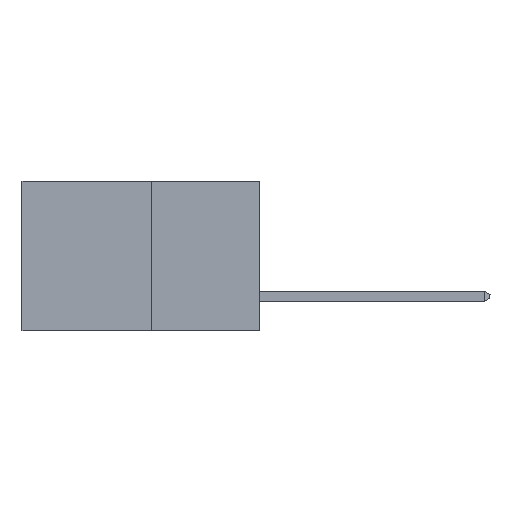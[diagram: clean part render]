
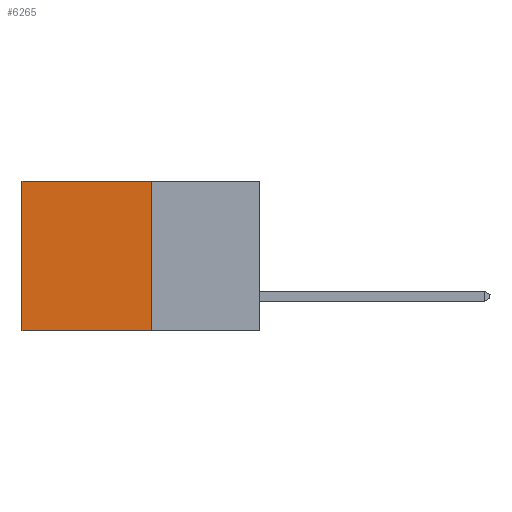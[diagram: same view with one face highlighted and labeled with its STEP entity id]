
A CAD part, left-side view. The second image highlights one B-rep face of the part: STEP entity #6265.
In plain terms, the highlighted planar face has unit normal (-1, 0, 0).
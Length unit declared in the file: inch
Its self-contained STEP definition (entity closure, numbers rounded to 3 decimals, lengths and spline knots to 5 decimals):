
#928 = CARTESIAN_POINT ( 'NONE',  ( 0.277, 0.59, -0.37 ) ) ;
#1916 = CARTESIAN_POINT ( 'NONE',  ( 0.277, 0.59, -0.37 ) ) ;
#2006 = ORIENTED_EDGE ( 'NONE', *, *, #17416, .F. ) ;
#2059 = PLANE ( 'NONE',  #2698 ) ;
#2162 = CARTESIAN_POINT ( 'NONE',  ( 0.277, 0.27, -0.37 ) ) ;
#2698 = AXIS2_PLACEMENT_3D ( 'NONE', #19131, #6349, #21233 ) ;
#3882 = VECTOR ( 'NONE', #4320, 39.37008 ) ;
#3923 = ORIENTED_EDGE ( 'NONE', *, *, #12436, .T. ) ;
#3998 = DIRECTION ( 'NONE',  ( 0., 1., 0. ) ) ;
#4320 = DIRECTION ( 'NONE',  ( 0., 0., -1. ) ) ;
#5439 = VERTEX_POINT ( 'NONE', #22619 ) ;
#6265 = ADVANCED_FACE ( 'NONE', ( #14561 ), #2059, .F. ) ;
#6349 = DIRECTION ( 'NONE',  ( 1., 0., 0. ) ) ;
#7145 = EDGE_LOOP ( 'NONE', ( #3923, #24545, #2006, #20848 ) ) ;
#8177 = CARTESIAN_POINT ( 'NONE',  ( 0.277, 0.27, 0. ) ) ;
#9681 = DIRECTION ( 'NONE',  ( 0., 1., 0. ) ) ;
#11301 = CARTESIAN_POINT ( 'NONE',  ( 0.277, 0.27, -0.37 ) ) ;
#12436 = EDGE_CURVE ( 'NONE', #5439, #22808, #20549, .T. ) ;
#12644 = DIRECTION ( 'NONE',  ( 0., 0., -1. ) ) ;
#12899 = VECTOR ( 'NONE', #3998, 39.37008 ) ;
#14236 = LINE ( 'NONE', #8177, #12899 ) ;
#14561 = FACE_OUTER_BOUND ( 'NONE', #7145, .T. ) ;
#15920 = LINE ( 'NONE', #2162, #3882 ) ;
#15949 = VERTEX_POINT ( 'NONE', #11301 ) ;
#16820 = EDGE_CURVE ( 'NONE', #15949, #22808, #19941, .T. ) ;
#17416 = EDGE_CURVE ( 'NONE', #23918, #15949, #15920, .T. ) ;
#18614 = VECTOR ( 'NONE', #9681, 39.37008 ) ;
#19131 = CARTESIAN_POINT ( 'NONE',  ( 0.277, 0.27, -0.37 ) ) ;
#19941 = LINE ( 'NONE', #24483, #18614 ) ;
#20273 = CARTESIAN_POINT ( 'NONE',  ( 0.277, 0.27, 0. ) ) ;
#20549 = LINE ( 'NONE', #1916, #21213 ) ;
#20848 = ORIENTED_EDGE ( 'NONE', *, *, #23059, .T. ) ;
#21213 = VECTOR ( 'NONE', #12644, 39.37008 ) ;
#21233 = DIRECTION ( 'NONE',  ( 0., 0., -1. ) ) ;
#22619 = CARTESIAN_POINT ( 'NONE',  ( 0.277, 0.59, 0. ) ) ;
#22808 = VERTEX_POINT ( 'NONE', #928 ) ;
#23059 = EDGE_CURVE ( 'NONE', #23918, #5439, #14236, .T. ) ;
#23918 = VERTEX_POINT ( 'NONE', #20273 ) ;
#24483 = CARTESIAN_POINT ( 'NONE',  ( 0.277, 0.27, -0.37 ) ) ;
#24545 = ORIENTED_EDGE ( 'NONE', *, *, #16820, .F. ) ;
